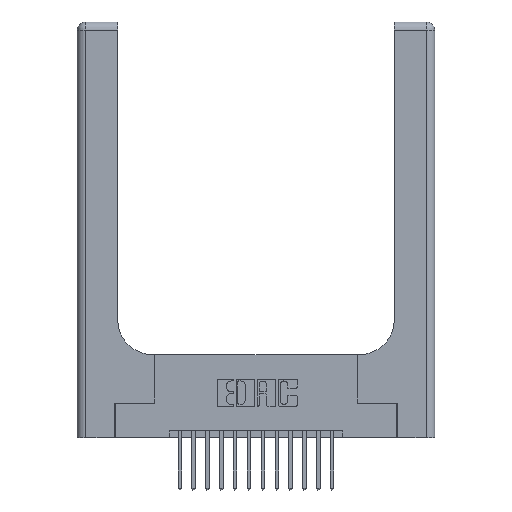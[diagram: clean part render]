
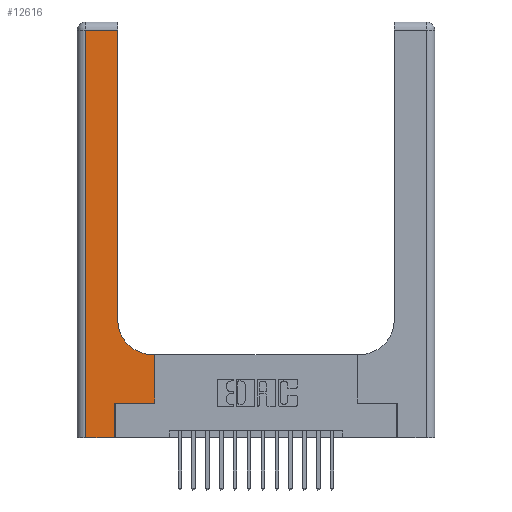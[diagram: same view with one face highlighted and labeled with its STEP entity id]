
A CAD part, top view. The second image highlights one B-rep face of the part: STEP entity #12616.
In plain terms, the highlighted planar face has unit normal (0, 0, 1).
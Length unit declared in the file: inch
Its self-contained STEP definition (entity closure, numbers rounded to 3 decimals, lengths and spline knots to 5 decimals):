
#27 = ORIENTED_EDGE ( 'NONE', *, *, #9960, .T. ) ;
#52 = LINE ( 'NONE', #10037, #15008 ) ;
#819 = LINE ( 'NONE', #2652, #12382 ) ;
#852 = CARTESIAN_POINT ( 'NONE',  ( 0.5415, 0.6, 0.37 ) ) ;
#1187 = ORIENTED_EDGE ( 'NONE', *, *, #17368, .T. ) ;
#1288 = AXIS2_PLACEMENT_3D ( 'NONE', #14814, #6222, #16238 ) ;
#1317 = AXIS2_PLACEMENT_3D ( 'NONE', #8643, #18666, #10137 ) ;
#1756 = CARTESIAN_POINT ( 'NONE',  ( 0.269, 0.25, 0.37 ) ) ;
#2264 = VERTEX_POINT ( 'NONE', #18615 ) ;
#2390 = CARTESIAN_POINT ( 'NONE',  ( 0.2915, 0.6, 0.37 ) ) ;
#2652 = CARTESIAN_POINT ( 'NONE',  ( 0.2915, 3., 0.37 ) ) ;
#3539 = ORIENTED_EDGE ( 'NONE', *, *, #17133, .T. ) ;
#3987 = CARTESIAN_POINT ( 'NONE',  ( 0.06, 3., 0.37 ) ) ;
#4109 = DIRECTION ( 'NONE',  ( 0., 1., 0. ) ) ;
#4143 = VECTOR ( 'NONE', #10220, 39.37008 ) ;
#4576 = CARTESIAN_POINT ( 'NONE',  ( 0.5585, 0.6, 0.37 ) ) ;
#4586 = VERTEX_POINT ( 'NONE', #5420 ) ;
#4646 = CARTESIAN_POINT ( 'NONE',  ( 0.06, 0., 0.37 ) ) ;
#5420 = CARTESIAN_POINT ( 'NONE',  ( 0.269, 0., 0.37 ) ) ;
#5479 = DIRECTION ( 'NONE',  ( 0., -1., 0. ) ) ;
#5515 = EDGE_CURVE ( 'NONE', #4586, #9344, #16064, .T. ) ;
#5648 = LINE ( 'NONE', #2390, #12810 ) ;
#6067 = CARTESIAN_POINT ( 'NONE',  ( 0.269, 0.25, 0.37 ) ) ;
#6157 = EDGE_LOOP ( 'NONE', ( #16024, #17863, #3539, #1187, #11453, #7295, #6751, #7224, #27 ) ) ;
#6222 = DIRECTION ( 'NONE',  ( 0., 0., -1. ) ) ;
#6625 = VECTOR ( 'NONE', #14917, 39.37008 ) ;
#6751 = ORIENTED_EDGE ( 'NONE', *, *, #14981, .T. ) ;
#6767 = VECTOR ( 'NONE', #17244, 39.37008 ) ;
#6864 = LINE ( 'NONE', #3987, #17383 ) ;
#7019 = FACE_OUTER_BOUND ( 'NONE', #6157, .T. ) ;
#7224 = ORIENTED_EDGE ( 'NONE', *, *, #8536, .T. ) ;
#7295 = ORIENTED_EDGE ( 'NONE', *, *, #8230, .T. ) ;
#8221 = VERTEX_POINT ( 'NONE', #4646 ) ;
#8230 = EDGE_CURVE ( 'NONE', #9344, #13480, #10614, .T. ) ;
#8482 = VERTEX_POINT ( 'NONE', #852 ) ;
#8536 = EDGE_CURVE ( 'NONE', #14401, #8482, #5648, .T. ) ;
#8642 = EDGE_CURVE ( 'NONE', #2264, #18559, #819, .T. ) ;
#8643 = CARTESIAN_POINT ( 'NONE',  ( 0., 3., 0.37 ) ) ;
#8707 = PLANE ( 'NONE',  #1317 ) ;
#8725 = EDGE_CURVE ( 'NONE', #18559, #10658, #10596, .T. ) ;
#8797 = CARTESIAN_POINT ( 'NONE',  ( 0.269, 0., 0.37 ) ) ;
#9344 = VERTEX_POINT ( 'NONE', #6067 ) ;
#9960 = EDGE_CURVE ( 'NONE', #8482, #2264, #18148, .T. ) ;
#10037 = CARTESIAN_POINT ( 'NONE',  ( 0.5585, 0.25, 0.37 ) ) ;
#10137 = DIRECTION ( 'NONE',  ( -1., 0., 0. ) ) ;
#10220 = DIRECTION ( 'NONE',  ( 0., 1., 0. ) ) ;
#10444 = DIRECTION ( 'NONE',  ( 1., 0., 0. ) ) ;
#10596 = LINE ( 'NONE', #15800, #6767 ) ;
#10614 = LINE ( 'NONE', #1756, #18180 ) ;
#10658 = VERTEX_POINT ( 'NONE', #16218 ) ;
#11453 = ORIENTED_EDGE ( 'NONE', *, *, #5515, .T. ) ;
#12046 = CARTESIAN_POINT ( 'NONE',  ( 0.5585, 0.25, 0.37 ) ) ;
#12382 = VECTOR ( 'NONE', #4109, 39.37008 ) ;
#12552 = DIRECTION ( 'NONE',  ( -1., 0., 0. ) ) ;
#12616 = ADVANCED_FACE ( 'NONE', ( #7019 ), #8707, .F. ) ;
#12810 = VECTOR ( 'NONE', #12552, 39.37008 ) ;
#13480 = VERTEX_POINT ( 'NONE', #12046 ) ;
#14338 = DIRECTION ( 'NONE',  ( 0., 1., 0. ) ) ;
#14401 = VERTEX_POINT ( 'NONE', #4576 ) ;
#14814 = CARTESIAN_POINT ( 'NONE',  ( 0.5415, 0.85, 0.37 ) ) ;
#14917 = DIRECTION ( 'NONE',  ( 1., 0., 0. ) ) ;
#14981 = EDGE_CURVE ( 'NONE', #13480, #14401, #52, .T. ) ;
#15008 = VECTOR ( 'NONE', #14338, 39.37008 ) ;
#15800 = CARTESIAN_POINT ( 'NONE',  ( 0., 2.94, 0.37 ) ) ;
#16024 = ORIENTED_EDGE ( 'NONE', *, *, #8642, .T. ) ;
#16064 = LINE ( 'NONE', #8797, #4143 ) ;
#16174 = CARTESIAN_POINT ( 'NONE',  ( 0.2915, 2.94, 0.37 ) ) ;
#16218 = CARTESIAN_POINT ( 'NONE',  ( 0.06, 2.94, 0.37 ) ) ;
#16238 = DIRECTION ( 'NONE',  ( 1., 0., 0. ) ) ;
#16337 = CARTESIAN_POINT ( 'NONE',  ( 0., 0., 0.37 ) ) ;
#17133 = EDGE_CURVE ( 'NONE', #10658, #8221, #6864, .T. ) ;
#17244 = DIRECTION ( 'NONE',  ( -1., 0., 0. ) ) ;
#17368 = EDGE_CURVE ( 'NONE', #8221, #4586, #18039, .T. ) ;
#17383 = VECTOR ( 'NONE', #5479, 39.37008 ) ;
#17863 = ORIENTED_EDGE ( 'NONE', *, *, #8725, .T. ) ;
#18039 = LINE ( 'NONE', #16337, #6625 ) ;
#18148 = CIRCLE ( 'NONE', #1288, 0.25 ) ;
#18180 = VECTOR ( 'NONE', #10444, 39.37008 ) ;
#18559 = VERTEX_POINT ( 'NONE', #16174 ) ;
#18615 = CARTESIAN_POINT ( 'NONE',  ( 0.2915, 0.85, 0.37 ) ) ;
#18666 = DIRECTION ( 'NONE',  ( 0., 0., -1. ) ) ;
